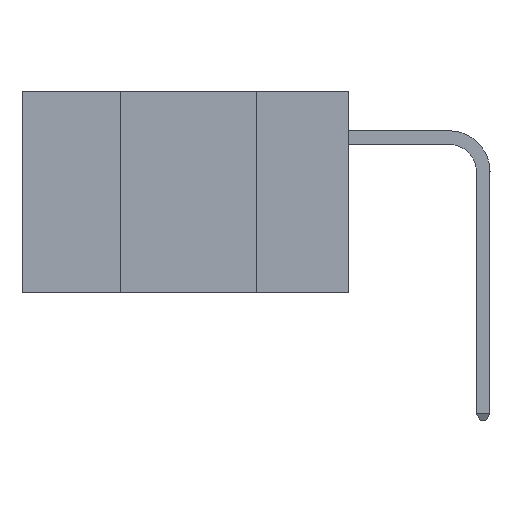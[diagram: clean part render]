
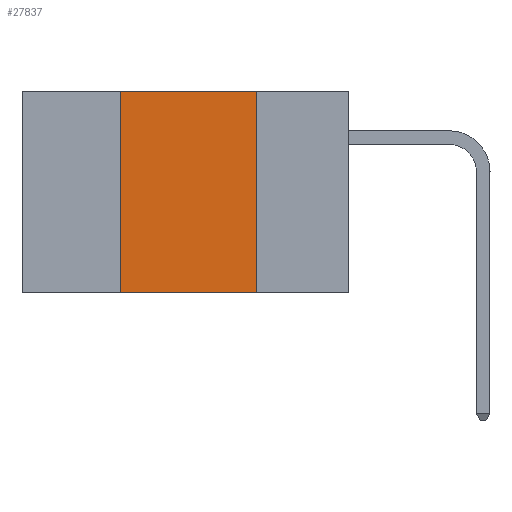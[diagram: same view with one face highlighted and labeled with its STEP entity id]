
A CAD part, left-side view. The second image highlights one B-rep face of the part: STEP entity #27837.
In plain terms, the highlighted planar face has unit normal (-1, 0, 0).
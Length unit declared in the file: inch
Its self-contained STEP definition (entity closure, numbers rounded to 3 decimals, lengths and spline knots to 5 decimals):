
#793 = VERTEX_POINT ( 'NONE', #20340 ) ;
#885 = CARTESIAN_POINT ( 'NONE',  ( 0., 0.17, 0. ) ) ;
#2210 = VERTEX_POINT ( 'NONE', #35614 ) ;
#2805 = ORIENTED_EDGE ( 'NONE', *, *, #7637, .F. ) ;
#3477 = CARTESIAN_POINT ( 'NONE',  ( 0., 0.6, 0. ) ) ;
#3787 = CARTESIAN_POINT ( 'NONE',  ( 0., 0.6, -0.37 ) ) ;
#5319 = DIRECTION ( 'NONE',  ( 0., 0., -1. ) ) ;
#5499 = VERTEX_POINT ( 'NONE', #885 ) ;
#6678 = DIRECTION ( 'NONE',  ( 0., 0., 1. ) ) ;
#7637 = EDGE_CURVE ( 'NONE', #37824, #793, #12304, .T. ) ;
#9584 = FACE_OUTER_BOUND ( 'NONE', #35209, .T. ) ;
#10053 = EDGE_CURVE ( 'NONE', #793, #5499, #28371, .T. ) ;
#12304 = LINE ( 'NONE', #19280, #27156 ) ;
#13623 = LINE ( 'NONE', #18326, #17572 ) ;
#17572 = VECTOR ( 'NONE', #5319, 39.37008 ) ;
#18326 = CARTESIAN_POINT ( 'NONE',  ( 0., 0.17, 0. ) ) ;
#18789 = ORIENTED_EDGE ( 'NONE', *, *, #10053, .F. ) ;
#19280 = CARTESIAN_POINT ( 'NONE',  ( 0., 0.42, 0. ) ) ;
#19363 = DIRECTION ( 'NONE',  ( 0., -1., 0. ) ) ;
#20155 = AXIS2_PLACEMENT_3D ( 'NONE', #3477, #29250, #32028 ) ;
#20340 = CARTESIAN_POINT ( 'NONE',  ( 0., 0.42, 0. ) ) ;
#22791 = CARTESIAN_POINT ( 'NONE',  ( 0., 0.42, -0.37 ) ) ;
#22828 = CARTESIAN_POINT ( 'NONE',  ( 0., 0.6, 0. ) ) ;
#25690 = DIRECTION ( 'NONE',  ( 0., -1., 0. ) ) ;
#27156 = VECTOR ( 'NONE', #6678, 39.37008 ) ;
#27371 = ORIENTED_EDGE ( 'NONE', *, *, #34398, .T. ) ;
#27837 = ADVANCED_FACE ( 'NONE', ( #9584 ), #28831, .F. ) ;
#27887 = ORIENTED_EDGE ( 'NONE', *, *, #38161, .F. ) ;
#28371 = LINE ( 'NONE', #22828, #37304 ) ;
#28502 = LINE ( 'NONE', #3787, #29009 ) ;
#28831 = PLANE ( 'NONE',  #20155 ) ;
#29009 = VECTOR ( 'NONE', #25690, 39.37008 ) ;
#29250 = DIRECTION ( 'NONE',  ( 1., 0., 0. ) ) ;
#32028 = DIRECTION ( 'NONE',  ( 0., 0., -1. ) ) ;
#34398 = EDGE_CURVE ( 'NONE', #37824, #2210, #28502, .T. ) ;
#35209 = EDGE_LOOP ( 'NONE', ( #27887, #18789, #2805, #27371 ) ) ;
#35614 = CARTESIAN_POINT ( 'NONE',  ( 0., 0.17, -0.37 ) ) ;
#37304 = VECTOR ( 'NONE', #19363, 39.37008 ) ;
#37824 = VERTEX_POINT ( 'NONE', #22791 ) ;
#38161 = EDGE_CURVE ( 'NONE', #5499, #2210, #13623, .T. ) ;
